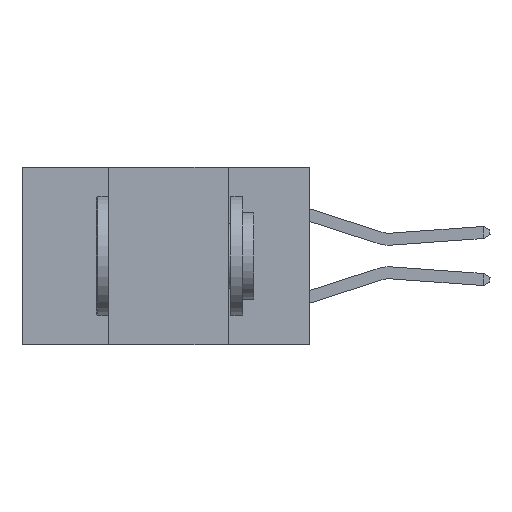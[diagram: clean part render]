
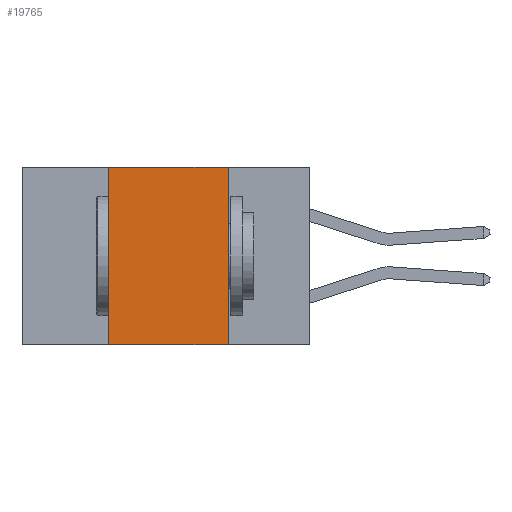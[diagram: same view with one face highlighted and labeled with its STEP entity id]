
A CAD part, left-side view. The second image highlights one B-rep face of the part: STEP entity #19765.
In plain terms, the highlighted planar face has unit normal (-1, 0, 0).
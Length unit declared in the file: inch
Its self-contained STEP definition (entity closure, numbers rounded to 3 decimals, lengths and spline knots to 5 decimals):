
#126 = CARTESIAN_POINT ( 'NONE',  ( 0., 0.42, -0.37 ) ) ;
#182 = DIRECTION ( 'NONE',  ( 0., -1., 0. ) ) ;
#253 = VERTEX_POINT ( 'NONE', #126 ) ;
#952 = ORIENTED_EDGE ( 'NONE', *, *, #16696, .T. ) ;
#1289 = VECTOR ( 'NONE', #26164, 39.37008 ) ;
#1641 = LINE ( 'NONE', #28465, #16221 ) ;
#1782 = CARTESIAN_POINT ( 'NONE',  ( 0., 0.42, 0. ) ) ;
#2648 = CARTESIAN_POINT ( 'NONE',  ( 0., 0.42, 0. ) ) ;
#2908 = EDGE_CURVE ( 'NONE', #21908, #9229, #18203, .T. ) ;
#4351 = VERTEX_POINT ( 'NONE', #1782 ) ;
#5396 = LINE ( 'NONE', #19133, #1289 ) ;
#6947 = CARTESIAN_POINT ( 'NONE',  ( 0., 0.17, -0.37 ) ) ;
#7246 = EDGE_LOOP ( 'NONE', ( #7890, #30183, #13365, #952 ) ) ;
#7890 = ORIENTED_EDGE ( 'NONE', *, *, #2908, .F. ) ;
#8971 = CARTESIAN_POINT ( 'NONE',  ( 0., 0.17, 0. ) ) ;
#9229 = VERTEX_POINT ( 'NONE', #6947 ) ;
#10416 = EDGE_CURVE ( 'NONE', #253, #4351, #11454, .T. ) ;
#11454 = LINE ( 'NONE', #2648, #16268 ) ;
#12117 = DIRECTION ( 'NONE',  ( 1., 0., 0. ) ) ;
#12194 = DIRECTION ( 'NONE',  ( 0., 0., 1. ) ) ;
#13365 = ORIENTED_EDGE ( 'NONE', *, *, #10416, .F. ) ;
#13506 = AXIS2_PLACEMENT_3D ( 'NONE', #17570, #12117, #14492 ) ;
#14492 = DIRECTION ( 'NONE',  ( 0., 0., -1. ) ) ;
#15609 = FACE_OUTER_BOUND ( 'NONE', #7246, .T. ) ;
#16221 = VECTOR ( 'NONE', #182, 39.37008 ) ;
#16268 = VECTOR ( 'NONE', #12194, 39.37008 ) ;
#16696 = EDGE_CURVE ( 'NONE', #253, #9229, #5396, .T. ) ;
#16853 = PLANE ( 'NONE',  #13506 ) ;
#17570 = CARTESIAN_POINT ( 'NONE',  ( 0., 0.6, 0. ) ) ;
#18121 = DIRECTION ( 'NONE',  ( 0., 0., -1. ) ) ;
#18203 = LINE ( 'NONE', #8971, #28320 ) ;
#19133 = CARTESIAN_POINT ( 'NONE',  ( 0., 0.6, -0.37 ) ) ;
#19765 = ADVANCED_FACE ( 'NONE', ( #15609 ), #16853, .F. ) ;
#21908 = VERTEX_POINT ( 'NONE', #29515 ) ;
#24106 = EDGE_CURVE ( 'NONE', #4351, #21908, #1641, .T. ) ;
#26164 = DIRECTION ( 'NONE',  ( 0., -1., 0. ) ) ;
#28320 = VECTOR ( 'NONE', #18121, 39.37008 ) ;
#28465 = CARTESIAN_POINT ( 'NONE',  ( 0., 0.6, 0. ) ) ;
#29515 = CARTESIAN_POINT ( 'NONE',  ( 0., 0.17, 0. ) ) ;
#30183 = ORIENTED_EDGE ( 'NONE', *, *, #24106, .F. ) ;
